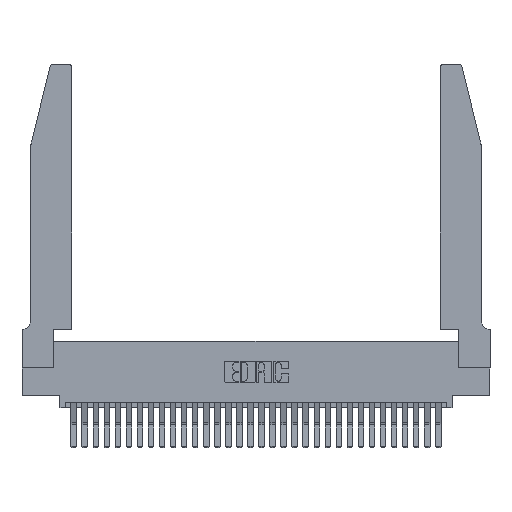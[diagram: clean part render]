
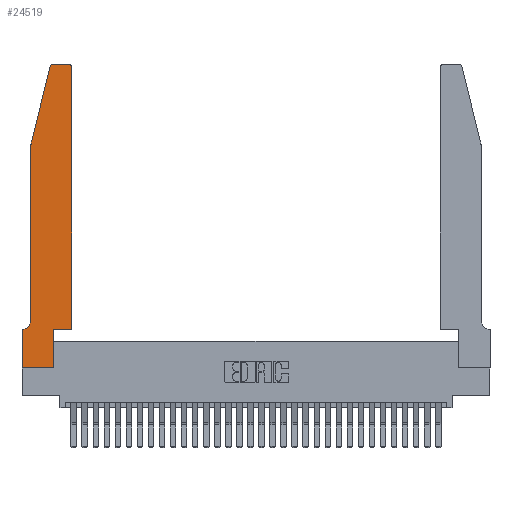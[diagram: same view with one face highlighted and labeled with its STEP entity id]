
A CAD part, top view. The second image highlights one B-rep face of the part: STEP entity #24519.
In plain terms, the highlighted planar face has unit normal (0, 0, 1).
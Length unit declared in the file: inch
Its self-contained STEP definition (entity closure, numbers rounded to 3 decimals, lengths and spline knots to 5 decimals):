
#290 = LINE ( 'NONE', #31656, #29147 ) ;
#606 = VERTEX_POINT ( 'NONE', #30218 ) ;
#900 = ORIENTED_EDGE ( 'NONE', *, *, #29400, .T. ) ;
#1141 = EDGE_CURVE ( 'NONE', #606, #7141, #2768, .T. ) ;
#2299 = EDGE_CURVE ( 'NONE', #20957, #6585, #290, .T. ) ;
#2339 = LINE ( 'NONE', #17725, #3907 ) ;
#2768 = LINE ( 'NONE', #28223, #21765 ) ;
#3157 = VERTEX_POINT ( 'NONE', #24944 ) ;
#3447 = DIRECTION ( 'NONE',  ( 0., 0., 1. ) ) ;
#3907 = VECTOR ( 'NONE', #25321, 39.37008 ) ;
#4060 = VECTOR ( 'NONE', #28440, 39.37008 ) ;
#4095 = DIRECTION ( 'NONE',  ( 1., 0., 0. ) ) ;
#4544 = EDGE_CURVE ( 'NONE', #28747, #12063, #5925, .T. ) ;
#5236 = ORIENTED_EDGE ( 'NONE', *, *, #16012, .T. ) ;
#5768 = CARTESIAN_POINT ( 'NONE',  ( 0.0755, 2., 0.37 ) ) ;
#5925 = LINE ( 'NONE', #28728, #19407 ) ;
#6585 = VERTEX_POINT ( 'NONE', #7937 ) ;
#6988 = VERTEX_POINT ( 'NONE', #32440 ) ;
#7141 = VERTEX_POINT ( 'NONE', #20544 ) ;
#7499 = DIRECTION ( 'NONE',  ( 0., 0., 1. ) ) ;
#7643 = VERTEX_POINT ( 'NONE', #23548 ) ;
#7717 = VECTOR ( 'NONE', #15519, 39.37008 ) ;
#7915 = EDGE_CURVE ( 'NONE', #22312, #6988, #19594, .T. ) ;
#7937 = CARTESIAN_POINT ( 'NONE',  ( 0.0755, 2., 0.37 ) ) ;
#9203 = AXIS2_PLACEMENT_3D ( 'NONE', #11887, #3447, #4095 ) ;
#9551 = ORIENTED_EDGE ( 'NONE', *, *, #1141, .T. ) ;
#9595 = ORIENTED_EDGE ( 'NONE', *, *, #13954, .T. ) ;
#9716 = LINE ( 'NONE', #20248, #11740 ) ;
#9949 = CARTESIAN_POINT ( 'NONE',  ( 0.4205, 2.75, 0.37 ) ) ;
#10731 = CARTESIAN_POINT ( 'NONE',  ( 0.2605, 2.75, 0.37 ) ) ;
#10964 = DIRECTION ( 'NONE',  ( 0., 0., -1. ) ) ;
#11065 = CIRCLE ( 'NONE', #22149, 0.07 ) ;
#11319 = ORIENTED_EDGE ( 'NONE', *, *, #23197, .T. ) ;
#11680 = ORIENTED_EDGE ( 'NONE', *, *, #14428, .T. ) ;
#11740 = VECTOR ( 'NONE', #17935, 39.37008 ) ;
#11833 = CARTESIAN_POINT ( 'NONE',  ( 0., 0.35, 0.37 ) ) ;
#11887 = CARTESIAN_POINT ( 'NONE',  ( 0.284, 2.72, 0.37 ) ) ;
#12063 = VERTEX_POINT ( 'NONE', #11833 ) ;
#12507 = DIRECTION ( 'NONE',  ( 1., 0., 0. ) ) ;
#13766 = DIRECTION ( 'NONE',  ( -1., 0., 0. ) ) ;
#13954 = EDGE_CURVE ( 'NONE', #3157, #25281, #2339, .T. ) ;
#13975 = CARTESIAN_POINT ( 'NONE',  ( 0.4505, 0.35, 0.37 ) ) ;
#14035 = DIRECTION ( 'NONE',  ( -0.239, -0.971, 0. ) ) ;
#14428 = EDGE_CURVE ( 'NONE', #32600, #28747, #11065, .T. ) ;
#15099 = LINE ( 'NONE', #13975, #21415 ) ;
#15137 = LINE ( 'NONE', #5768, #23396 ) ;
#15519 = DIRECTION ( 'NONE',  ( -1., 0., 0. ) ) ;
#16012 = EDGE_CURVE ( 'NONE', #25281, #606, #15099, .T. ) ;
#16050 = ORIENTED_EDGE ( 'NONE', *, *, #2299, .T. ) ;
#16288 = CARTESIAN_POINT ( 'NONE',  ( 0.0755, 0.42, 0.37 ) ) ;
#16614 = DIRECTION ( 'NONE',  ( 1., 0., 0. ) ) ;
#16743 = AXIS2_PLACEMENT_3D ( 'NONE', #25175, #27580, #12507 ) ;
#16952 = ORIENTED_EDGE ( 'NONE', *, *, #4544, .T. ) ;
#17725 = CARTESIAN_POINT ( 'NONE',  ( 0.2865, 0.35, 0.37 ) ) ;
#17935 = DIRECTION ( 'NONE',  ( 1., 0., 0. ) ) ;
#18612 = DIRECTION ( 'NONE',  ( 0., -1., 0. ) ) ;
#19274 = EDGE_CURVE ( 'NONE', #6585, #32600, #15137, .T. ) ;
#19407 = VECTOR ( 'NONE', #13766, 39.37008 ) ;
#19512 = ORIENTED_EDGE ( 'NONE', *, *, #7915, .T. ) ;
#19594 = LINE ( 'NONE', #10731, #7717 ) ;
#19855 = CARTESIAN_POINT ( 'NONE',  ( 0.25487, 2.72718, 0.37 ) ) ;
#20086 = EDGE_LOOP ( 'NONE', ( #19512, #11319, #16050, #26769, #11680, #16952, #21102, #20140, #9595, #5236, #9551, #900 ) ) ;
#20140 = ORIENTED_EDGE ( 'NONE', *, *, #24456, .T. ) ;
#20248 = CARTESIAN_POINT ( 'NONE',  ( 0., 0., 0.37 ) ) ;
#20544 = CARTESIAN_POINT ( 'NONE',  ( 0.4505, 2.72, 0.37 ) ) ;
#20546 = CARTESIAN_POINT ( 'NONE',  ( 0.2865, 0.35, 0.37 ) ) ;
#20918 = CIRCLE ( 'NONE', #16743, 0.03 ) ;
#20957 = VERTEX_POINT ( 'NONE', #19855 ) ;
#21102 = ORIENTED_EDGE ( 'NONE', *, *, #30810, .T. ) ;
#21122 = LINE ( 'NONE', #26339, #4060 ) ;
#21415 = VECTOR ( 'NONE', #16614, 39.37008 ) ;
#21567 = DIRECTION ( 'NONE',  ( -1., 0., 0. ) ) ;
#21765 = VECTOR ( 'NONE', #30793, 39.37008 ) ;
#22149 = AXIS2_PLACEMENT_3D ( 'NONE', #26171, #10964, #21567 ) ;
#22312 = VERTEX_POINT ( 'NONE', #9949 ) ;
#22692 = CARTESIAN_POINT ( 'NONE',  ( 0., 0.35, 0.37 ) ) ;
#23197 = EDGE_CURVE ( 'NONE', #6988, #20957, #24384, .T. ) ;
#23396 = VECTOR ( 'NONE', #18612, 39.37008 ) ;
#23548 = CARTESIAN_POINT ( 'NONE',  ( 0., 0., 0.37 ) ) ;
#24357 = FACE_OUTER_BOUND ( 'NONE', #20086, .T. ) ;
#24384 = CIRCLE ( 'NONE', #9203, 0.03 ) ;
#24456 = EDGE_CURVE ( 'NONE', #7643, #3157, #9716, .T. ) ;
#24519 = ADVANCED_FACE ( 'NONE', ( #24357 ), #28061, .T. ) ;
#24944 = CARTESIAN_POINT ( 'NONE',  ( 0.2865, 0., 0.37 ) ) ;
#25175 = CARTESIAN_POINT ( 'NONE',  ( 0.4205, 2.72, 0.37 ) ) ;
#25281 = VERTEX_POINT ( 'NONE', #20546 ) ;
#25321 = DIRECTION ( 'NONE',  ( 0., 1., 0. ) ) ;
#26171 = CARTESIAN_POINT ( 'NONE',  ( 0.0055, 0.42, 0.37 ) ) ;
#26339 = CARTESIAN_POINT ( 'NONE',  ( 0., 0., 0.37 ) ) ;
#26769 = ORIENTED_EDGE ( 'NONE', *, *, #19274, .T. ) ;
#27580 = DIRECTION ( 'NONE',  ( 0., 0., 1. ) ) ;
#27728 = DIRECTION ( 'NONE',  ( 1., 0., 0. ) ) ;
#28061 = PLANE ( 'NONE',  #29978 ) ;
#28223 = CARTESIAN_POINT ( 'NONE',  ( 0.4505, 0.35, 0.37 ) ) ;
#28440 = DIRECTION ( 'NONE',  ( 0., -1., 0. ) ) ;
#28728 = CARTESIAN_POINT ( 'NONE',  ( 0.0755, 0.35, 0.37 ) ) ;
#28747 = VERTEX_POINT ( 'NONE', #29626 ) ;
#29147 = VECTOR ( 'NONE', #14035, 39.37008 ) ;
#29400 = EDGE_CURVE ( 'NONE', #7141, #22312, #20918, .T. ) ;
#29626 = CARTESIAN_POINT ( 'NONE',  ( 0.0055, 0.35, 0.37 ) ) ;
#29978 = AXIS2_PLACEMENT_3D ( 'NONE', #22692, #7499, #27728 ) ;
#30218 = CARTESIAN_POINT ( 'NONE',  ( 0.4505, 0.35, 0.37 ) ) ;
#30793 = DIRECTION ( 'NONE',  ( 0., 1., 0. ) ) ;
#30810 = EDGE_CURVE ( 'NONE', #12063, #7643, #21122, .T. ) ;
#31656 = CARTESIAN_POINT ( 'NONE',  ( 0.0755, 2., 0.37 ) ) ;
#32440 = CARTESIAN_POINT ( 'NONE',  ( 0.284, 2.75, 0.37 ) ) ;
#32600 = VERTEX_POINT ( 'NONE', #16288 ) ;
